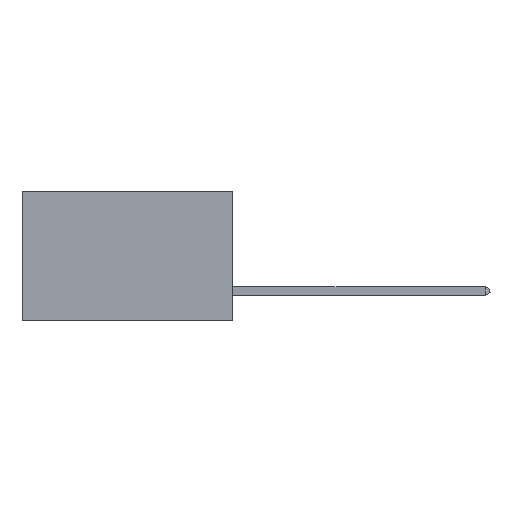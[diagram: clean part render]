
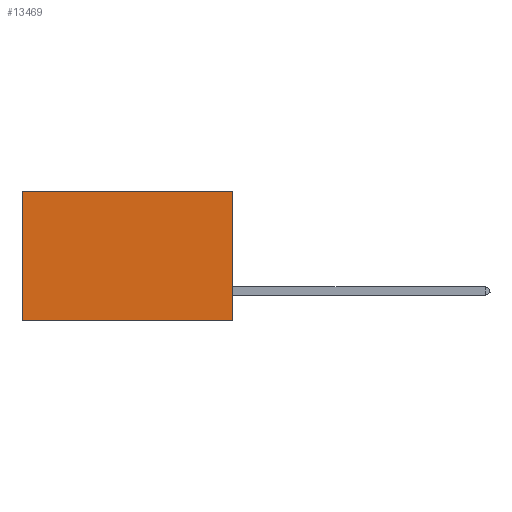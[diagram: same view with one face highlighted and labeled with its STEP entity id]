
A CAD part, left-side view. The second image highlights one B-rep face of the part: STEP entity #13469.
In plain terms, the highlighted planar face has unit normal (-1, 0, 0).
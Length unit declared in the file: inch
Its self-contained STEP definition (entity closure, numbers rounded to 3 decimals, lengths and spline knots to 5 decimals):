
#83 = DIRECTION ( 'NONE',  ( 0., 1., 0. ) ) ;
#250 = CARTESIAN_POINT ( 'NONE',  ( 0.2875, 0.6, 0. ) ) ;
#453 = AXIS2_PLACEMENT_3D ( 'NONE', #12361, #13589, #5982 ) ;
#1057 = ORIENTED_EDGE ( 'NONE', *, *, #3339, .F. ) ;
#1149 = LINE ( 'NONE', #12824, #12665 ) ;
#1184 = VERTEX_POINT ( 'NONE', #5246 ) ;
#1215 = CARTESIAN_POINT ( 'NONE',  ( 0.2875, 0., 0. ) ) ;
#2572 = VERTEX_POINT ( 'NONE', #12453 ) ;
#3200 = LINE ( 'NONE', #250, #11029 ) ;
#3238 = DIRECTION ( 'NONE',  ( 0., 0., -1. ) ) ;
#3339 = EDGE_CURVE ( 'NONE', #7914, #1184, #12180, .T. ) ;
#4955 = FACE_OUTER_BOUND ( 'NONE', #13359, .T. ) ;
#5246 = CARTESIAN_POINT ( 'NONE',  ( 0.2875, 0., -0.37 ) ) ;
#5261 = VECTOR ( 'NONE', #7540, 39.37008 ) ;
#5982 = DIRECTION ( 'NONE',  ( 0., 0., -1. ) ) ;
#6581 = LINE ( 'NONE', #11789, #5261 ) ;
#7089 = ORIENTED_EDGE ( 'NONE', *, *, #7666, .T. ) ;
#7540 = DIRECTION ( 'NONE',  ( 0., 1., 0. ) ) ;
#7666 = EDGE_CURVE ( 'NONE', #7914, #2572, #6581, .T. ) ;
#7735 = DIRECTION ( 'NONE',  ( 0., 0., -1. ) ) ;
#7914 = VERTEX_POINT ( 'NONE', #1215 ) ;
#8518 = PLANE ( 'NONE',  #453 ) ;
#8719 = CARTESIAN_POINT ( 'NONE',  ( 0.2875, 0., 0. ) ) ;
#9028 = ORIENTED_EDGE ( 'NONE', *, *, #13794, .F. ) ;
#9308 = VECTOR ( 'NONE', #3238, 39.37008 ) ;
#9865 = EDGE_CURVE ( 'NONE', #2572, #10499, #3200, .T. ) ;
#10360 = ORIENTED_EDGE ( 'NONE', *, *, #9865, .T. ) ;
#10499 = VERTEX_POINT ( 'NONE', #12931 ) ;
#11029 = VECTOR ( 'NONE', #7735, 39.37008 ) ;
#11789 = CARTESIAN_POINT ( 'NONE',  ( 0.2875, 0., 0. ) ) ;
#12180 = LINE ( 'NONE', #8719, #9308 ) ;
#12361 = CARTESIAN_POINT ( 'NONE',  ( 0.2875, 0., 0. ) ) ;
#12453 = CARTESIAN_POINT ( 'NONE',  ( 0.2875, 0.6, 0. ) ) ;
#12665 = VECTOR ( 'NONE', #83, 39.37008 ) ;
#12824 = CARTESIAN_POINT ( 'NONE',  ( 0.2875, 0., -0.37 ) ) ;
#12931 = CARTESIAN_POINT ( 'NONE',  ( 0.2875, 0.6, -0.37 ) ) ;
#13359 = EDGE_LOOP ( 'NONE', ( #10360, #9028, #1057, #7089 ) ) ;
#13469 = ADVANCED_FACE ( 'NONE', ( #4955 ), #8518, .F. ) ;
#13589 = DIRECTION ( 'NONE',  ( 1., 0., 0. ) ) ;
#13794 = EDGE_CURVE ( 'NONE', #1184, #10499, #1149, .T. ) ;
